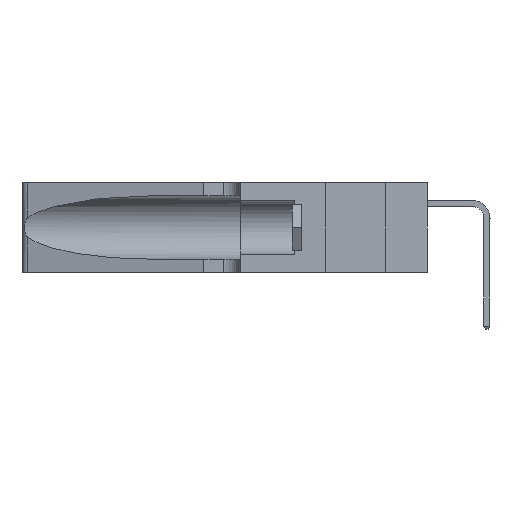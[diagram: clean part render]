
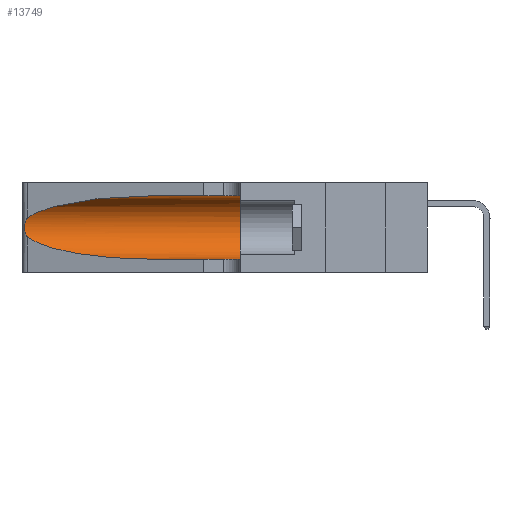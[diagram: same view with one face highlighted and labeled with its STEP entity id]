
A CAD part, left-side view. The second image highlights one B-rep face of the part: STEP entity #13749.
In plain terms, the highlighted cylindrical face has radius 3.308 mm (diameter 6.617 mm), a partial arc.
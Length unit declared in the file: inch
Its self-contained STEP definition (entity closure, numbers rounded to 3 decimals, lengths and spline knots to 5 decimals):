
#532 = DIRECTION ( 'NONE',  ( 0., -1., 0. ) ) ;
#2121 = CARTESIAN_POINT ( 'NONE',  ( 0.1305, 1.61858, 0.31525 ) ) ;
#2286 = ORIENTED_EDGE ( 'NONE', *, *, #17513, .T. ) ;
#3114 = CARTESIAN_POINT ( 'NONE',  ( 0.26075, 1.23896, 0.178 ) ) ;
#3811 = ORIENTED_EDGE ( 'NONE', *, *, #39231, .T. ) ;
#4582 = VECTOR ( 'NONE', #532, 39.37008 ) ;
#4730 = CARTESIAN_POINT ( 'NONE',  ( 0.1305, 0.72297, 0.31525 ) ) ;
#5740 = FACE_OUTER_BOUND ( 'NONE', #33604, .T. ) ;
#6544 = CARTESIAN_POINT ( 'NONE',  ( 0.25856, 1.23593, 0.16098 ) ) ;
#7494 = CIRCLE ( 'NONE', #39523, 0.13025 ) ;
#9083 = CARTESIAN_POINT ( 'NONE',  ( 0.18966, 0.96281, 0.05475 ) ) ;
#9253 = CARTESIAN_POINT ( 'NONE',  ( 0.1305, 0.35, 0.31525 ) ) ;
#9563 = CARTESIAN_POINT ( 'NONE',  ( 0.1305, 0.35, 0.185 ) ) ;
#9623 = CARTESIAN_POINT ( 'NONE',  ( 0.1305, 0.72297, 0.05475 ) ) ;
#9986 = CARTESIAN_POINT ( 'NONE',  ( 0.25639, 1.23186, 0.15144 ) ) ;
#10925 = LINE ( 'NONE', #2121, #18998 ) ;
#11566 = CARTESIAN_POINT ( 'NONE',  ( 0.1305, 0.72297, 0.31525 ) ) ;
#13013 = DIRECTION ( 'NONE',  ( 0., 0., 1. ) ) ;
#13456 = CARTESIAN_POINT ( 'NONE',  ( 0.25487, 1.22718, 0.14631 ) ) ;
#13720 = LINE ( 'NONE', #24531, #4582 ) ;
#13749 = ADVANCED_FACE ( 'NONE', ( #5740 ), #39039, .F. ) ;
#15024 = CARTESIAN_POINT ( 'NONE',  ( 0.25487, 1.22718, 0.22369 ) ) ;
#16762 = CARTESIAN_POINT ( 'NONE',  ( 0.25639, 1.23184, 0.21858 ) ) ;
#17513 = EDGE_CURVE ( 'NONE', #42577, #23956, #26952, .T. ) ;
#17647 = EDGE_CURVE ( 'NONE', #42577, #18414, #10925, .T. ) ;
#18414 = VERTEX_POINT ( 'NONE', #9253 ) ;
#18480 = ORIENTED_EDGE ( 'NONE', *, *, #31296, .T. ) ;
#18509 = EDGE_CURVE ( 'NONE', #23956, #29328, #18978, .T. ) ;
#18978 = B_SPLINE_CURVE_WITH_KNOTS ( 'NONE', 3,
 ( #33737, #37326, #16762, #40770, #20206, #44252, #23669, #3114, #27105, #6544, #30549, #9986, #34032, #13456 ),
 .UNSPECIFIED., .F., .F.,
 ( 4, 2, 2, 2, 2, 2, 4 ),
 ( 0., 0.00027, 0.00053, 0.00107, 0.0016, 0.00187, 0.00214 ),
 .UNSPECIFIED. ) ;
#18998 = VECTOR ( 'NONE', #29581, 39.37008 ) ;
#19763 = DIRECTION ( 'NONE',  ( 0., 0., -1. ) ) ;
#20206 = CARTESIAN_POINT ( 'NONE',  ( 0.25854, 1.2359, 0.20912 ) ) ;
#20681 = ORIENTED_EDGE ( 'NONE', *, *, #18509, .T. ) ;
#22751 = CARTESIAN_POINT ( 'NONE',  ( 0.2373, 1.15595, 0.08982 ) ) ;
#23669 = CARTESIAN_POINT ( 'NONE',  ( 0.26075, 1.23896, 0.19203 ) ) ;
#23956 = VERTEX_POINT ( 'NONE', #34974 ) ;
#24400 = ORIENTED_EDGE ( 'NONE', *, *, #42185, .F. ) ;
#24531 = CARTESIAN_POINT ( 'NONE',  ( 0.1305, 1.61858, 0.05475 ) ) ;
#25237 = CARTESIAN_POINT ( 'NONE',  ( 0.18966, 0.96281, 0.31525 ) ) ;
#26952 =( BOUNDED_CURVE ( )  B_SPLINE_CURVE ( 3, ( #11566, #25237, #38914, #15024 ),
 .UNSPECIFIED., .F., .F. ) 
 B_SPLINE_CURVE_WITH_KNOTS ( ( 4, 4 ),
 ( 1.5708, 2.84003 ),
 .UNSPECIFIED. ) 
 CURVE ( )  GEOMETRIC_REPRESENTATION_ITEM ( )  RATIONAL_B_SPLINE_CURVE ( ( 1., 0.87, 0.87, 1. ) ) 
 REPRESENTATION_ITEM ( '' )  );
#27100 = ORIENTED_EDGE ( 'NONE', *, *, #17647, .F. ) ;
#27105 = CARTESIAN_POINT ( 'NONE',  ( 0.26017, 1.23833, 0.17102 ) ) ;
#29328 = VERTEX_POINT ( 'NONE', #36275 ) ;
#29581 = DIRECTION ( 'NONE',  ( 0., -1., 0. ) ) ;
#30549 = CARTESIAN_POINT ( 'NONE',  ( 0.25789, 1.23486, 0.15765 ) ) ;
#31296 = EDGE_CURVE ( 'NONE', #29328, #33126, #31606, .T. ) ;
#31606 =( BOUNDED_CURVE ( )  B_SPLINE_CURVE ( 3, ( #43324, #22751, #9083, #33112 ),
 .UNSPECIFIED., .F., .F. ) 
 B_SPLINE_CURVE_WITH_KNOTS ( ( 4, 4 ),
 ( 3.44316, 4.71239 ),
 .UNSPECIFIED. ) 
 CURVE ( )  GEOMETRIC_REPRESENTATION_ITEM ( )  RATIONAL_B_SPLINE_CURVE ( ( 1., 0.87, 0.87, 1. ) ) 
 REPRESENTATION_ITEM ( '' )  );
#33112 = CARTESIAN_POINT ( 'NONE',  ( 0.1305, 0.72297, 0.05475 ) ) ;
#33126 = VERTEX_POINT ( 'NONE', #9623 ) ;
#33602 = DIRECTION ( 'NONE',  ( 0., 1., 0. ) ) ;
#33604 = EDGE_LOOP ( 'NONE', ( #2286, #20681, #18480, #3811, #24400, #27100 ) ) ;
#33737 = CARTESIAN_POINT ( 'NONE',  ( 0.25487, 1.22718, 0.22369 ) ) ;
#34032 = CARTESIAN_POINT ( 'NONE',  ( 0.25555, 1.22993, 0.14849 ) ) ;
#34974 = CARTESIAN_POINT ( 'NONE',  ( 0.25487, 1.22718, 0.22369 ) ) ;
#36275 = CARTESIAN_POINT ( 'NONE',  ( 0.25487, 1.22718, 0.14631 ) ) ;
#36879 = CARTESIAN_POINT ( 'NONE',  ( 0.1305, 1.61858, 0.185 ) ) ;
#36963 = AXIS2_PLACEMENT_3D ( 'NONE', #36879, #40322, #19763 ) ;
#37326 = CARTESIAN_POINT ( 'NONE',  ( 0.25555, 1.22994, 0.2215 ) ) ;
#37362 = VERTEX_POINT ( 'NONE', #43155 ) ;
#38914 = CARTESIAN_POINT ( 'NONE',  ( 0.2373, 1.15595, 0.28018 ) ) ;
#39039 = CYLINDRICAL_SURFACE ( 'NONE', #36963, 0.13025 ) ;
#39231 = EDGE_CURVE ( 'NONE', #33126, #37362, #13720, .T. ) ;
#39523 = AXIS2_PLACEMENT_3D ( 'NONE', #9563, #33602, #13013 ) ;
#40322 = DIRECTION ( 'NONE',  ( 0., -1., 0. ) ) ;
#40770 = CARTESIAN_POINT ( 'NONE',  ( 0.25787, 1.23484, 0.2124 ) ) ;
#42185 = EDGE_CURVE ( 'NONE', #18414, #37362, #7494, .T. ) ;
#42577 = VERTEX_POINT ( 'NONE', #4730 ) ;
#43155 = CARTESIAN_POINT ( 'NONE',  ( 0.1305, 0.35, 0.05475 ) ) ;
#43324 = CARTESIAN_POINT ( 'NONE',  ( 0.25487, 1.22718, 0.14631 ) ) ;
#44252 = CARTESIAN_POINT ( 'NONE',  ( 0.26018, 1.23835, 0.19895 ) ) ;
